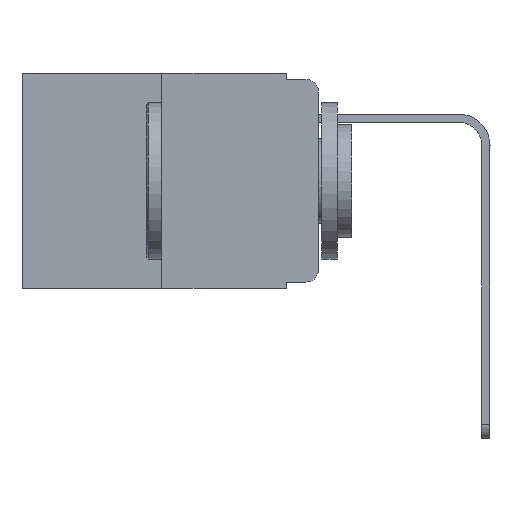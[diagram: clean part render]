
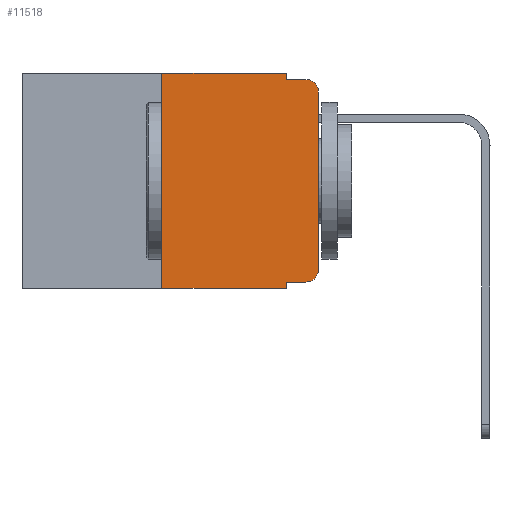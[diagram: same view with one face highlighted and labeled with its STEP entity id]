
A CAD part, left-side view. The second image highlights one B-rep face of the part: STEP entity #11518.
In plain terms, the highlighted planar face has unit normal (-1, 0, 0).
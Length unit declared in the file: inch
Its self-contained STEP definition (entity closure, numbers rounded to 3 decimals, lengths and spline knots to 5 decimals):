
#453 = CARTESIAN_POINT ( 'NONE',  ( 0., 0.473, 0. ) ) ;
#1000 = CARTESIAN_POINT ( 'NONE',  ( 0., 0.051, -0.01 ) ) ;
#1432 = PLANE ( 'NONE',  #17229 ) ;
#1486 = DIRECTION ( 'NONE',  ( 0., -1., 0. ) ) ;
#1608 = LINE ( 'NONE', #15582, #17619 ) ;
#2102 = DIRECTION ( 'NONE',  ( 0., 0., -1. ) ) ;
#2114 = AXIS2_PLACEMENT_3D ( 'NONE', #22359, #10714, #12764 ) ;
#2130 = VERTEX_POINT ( 'NONE', #12288 ) ;
#2171 = LINE ( 'NONE', #453, #10841 ) ;
#2318 = VECTOR ( 'NONE', #19342, 39.37008 ) ;
#3032 = CARTESIAN_POINT ( 'NONE',  ( 0., 0., -0.313 ) ) ;
#3380 = DIRECTION ( 'NONE',  ( 1., 0., 0. ) ) ;
#4158 = VECTOR ( 'NONE', #21739, 39.37008 ) ;
#4330 = CARTESIAN_POINT ( 'NONE',  ( 0., 0.02, -0.03 ) ) ;
#5041 = ORIENTED_EDGE ( 'NONE', *, *, #18230, .T. ) ;
#5197 = VECTOR ( 'NONE', #10844, 39.37008 ) ;
#6106 = EDGE_CURVE ( 'NONE', #11625, #12464, #2171, .T. ) ;
#6377 = ORIENTED_EDGE ( 'NONE', *, *, #21378, .F. ) ;
#7254 = ORIENTED_EDGE ( 'NONE', *, *, #9001, .F. ) ;
#7521 = CARTESIAN_POINT ( 'NONE',  ( 0., 0., 0. ) ) ;
#7698 = LINE ( 'NONE', #8960, #5197 ) ;
#8052 = CARTESIAN_POINT ( 'NONE',  ( 0., 0.25, -0.343 ) ) ;
#8109 = DIRECTION ( 'NONE',  ( 0., -1., 0. ) ) ;
#8110 = AXIS2_PLACEMENT_3D ( 'NONE', #4330, #19920, #2102 ) ;
#8438 = VERTEX_POINT ( 'NONE', #8052 ) ;
#8443 = CARTESIAN_POINT ( 'NONE',  ( 0., 0., -0.03 ) ) ;
#8870 = EDGE_CURVE ( 'NONE', #12464, #11852, #18313, .T. ) ;
#8960 = CARTESIAN_POINT ( 'NONE',  ( 0., 0.051, 0. ) ) ;
#9001 = EDGE_CURVE ( 'NONE', #11852, #16799, #24138, .T. ) ;
#9527 = LINE ( 'NONE', #14757, #24567 ) ;
#9677 = CARTESIAN_POINT ( 'NONE',  ( 0., 0.25, 0. ) ) ;
#10028 = LINE ( 'NONE', #19180, #19860 ) ;
#10051 = VERTEX_POINT ( 'NONE', #3032 ) ;
#10065 = LINE ( 'NONE', #7521, #2318 ) ;
#10714 = DIRECTION ( 'NONE',  ( -1., 0., 0. ) ) ;
#10841 = VECTOR ( 'NONE', #8109, 39.37008 ) ;
#10844 = DIRECTION ( 'NONE',  ( 0., 0., -1. ) ) ;
#10878 = CARTESIAN_POINT ( 'NONE',  ( 0., 0.051, -0.343 ) ) ;
#11312 = EDGE_CURVE ( 'NONE', #8438, #11625, #9527, .T. ) ;
#11518 = ADVANCED_FACE ( 'NONE', ( #20268 ), #1432, .F. ) ;
#11625 = VERTEX_POINT ( 'NONE', #9677 ) ;
#11852 = VERTEX_POINT ( 'NONE', #1000 ) ;
#12163 = CIRCLE ( 'NONE', #2114, 0.02 ) ;
#12288 = CARTESIAN_POINT ( 'NONE',  ( 0., 0.02, -0.333 ) ) ;
#12464 = VERTEX_POINT ( 'NONE', #24904 ) ;
#12764 = DIRECTION ( 'NONE',  ( 0., 0., -1. ) ) ;
#12777 = DIRECTION ( 'NONE',  ( 0., 0., 1. ) ) ;
#12886 = VERTEX_POINT ( 'NONE', #8443 ) ;
#14016 = VECTOR ( 'NONE', #25427, 39.37008 ) ;
#14424 = ORIENTED_EDGE ( 'NONE', *, *, #15403, .T. ) ;
#14757 = CARTESIAN_POINT ( 'NONE',  ( 0., 0.25, 0. ) ) ;
#15176 = CARTESIAN_POINT ( 'NONE',  ( 0., 0.473, 0. ) ) ;
#15403 = EDGE_CURVE ( 'NONE', #8438, #22575, #1608, .T. ) ;
#15582 = CARTESIAN_POINT ( 'NONE',  ( 0., 0.473, -0.343 ) ) ;
#15606 = CARTESIAN_POINT ( 'NONE',  ( 0., 0.02, -0.01 ) ) ;
#16799 = VERTEX_POINT ( 'NONE', #15606 ) ;
#17007 = EDGE_CURVE ( 'NONE', #2130, #10051, #12163, .T. ) ;
#17054 = ORIENTED_EDGE ( 'NONE', *, *, #11312, .F. ) ;
#17229 = AXIS2_PLACEMENT_3D ( 'NONE', #15176, #3380, #19126 ) ;
#17619 = VECTOR ( 'NONE', #23233, 39.37008 ) ;
#18136 = ORIENTED_EDGE ( 'NONE', *, *, #6106, .F. ) ;
#18230 = EDGE_CURVE ( 'NONE', #12886, #16799, #23769, .T. ) ;
#18313 = LINE ( 'NONE', #21827, #4158 ) ;
#19126 = DIRECTION ( 'NONE',  ( 0., 0., -1. ) ) ;
#19180 = CARTESIAN_POINT ( 'NONE',  ( 0., 0.051, -0.333 ) ) ;
#19342 = DIRECTION ( 'NONE',  ( 0., 0., 1. ) ) ;
#19672 = CARTESIAN_POINT ( 'NONE',  ( 0., 0.051, -0.333 ) ) ;
#19860 = VECTOR ( 'NONE', #1486, 39.37008 ) ;
#19920 = DIRECTION ( 'NONE',  ( -1., 0., 0. ) ) ;
#20169 = ORIENTED_EDGE ( 'NONE', *, *, #17007, .T. ) ;
#20268 = FACE_OUTER_BOUND ( 'NONE', #23848, .T. ) ;
#20720 = ORIENTED_EDGE ( 'NONE', *, *, #8870, .F. ) ;
#21378 = EDGE_CURVE ( 'NONE', #24628, #22575, #7698, .T. ) ;
#21578 = CARTESIAN_POINT ( 'NONE',  ( 0., 0.051, -0.01 ) ) ;
#21739 = DIRECTION ( 'NONE',  ( 0., 0., -1. ) ) ;
#21827 = CARTESIAN_POINT ( 'NONE',  ( 0., 0.051, 0. ) ) ;
#22359 = CARTESIAN_POINT ( 'NONE',  ( 0., 0.02, -0.313 ) ) ;
#22575 = VERTEX_POINT ( 'NONE', #10878 ) ;
#22628 = EDGE_CURVE ( 'NONE', #24628, #2130, #10028, .T. ) ;
#22742 = EDGE_CURVE ( 'NONE', #10051, #12886, #10065, .T. ) ;
#23233 = DIRECTION ( 'NONE',  ( 0., -1., 0. ) ) ;
#23691 = ORIENTED_EDGE ( 'NONE', *, *, #22628, .T. ) ;
#23769 = CIRCLE ( 'NONE', #8110, 0.02 ) ;
#23782 = ORIENTED_EDGE ( 'NONE', *, *, #22742, .T. ) ;
#23848 = EDGE_LOOP ( 'NONE', ( #23782, #5041, #7254, #20720, #18136, #17054, #14424, #6377, #23691, #20169 ) ) ;
#24138 = LINE ( 'NONE', #21578, #14016 ) ;
#24567 = VECTOR ( 'NONE', #12777, 39.37008 ) ;
#24628 = VERTEX_POINT ( 'NONE', #19672 ) ;
#24904 = CARTESIAN_POINT ( 'NONE',  ( 0., 0.051, 0. ) ) ;
#25427 = DIRECTION ( 'NONE',  ( 0., -1., 0. ) ) ;
